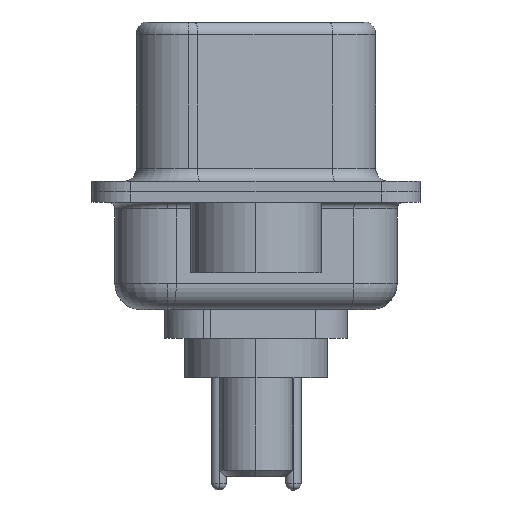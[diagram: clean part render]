
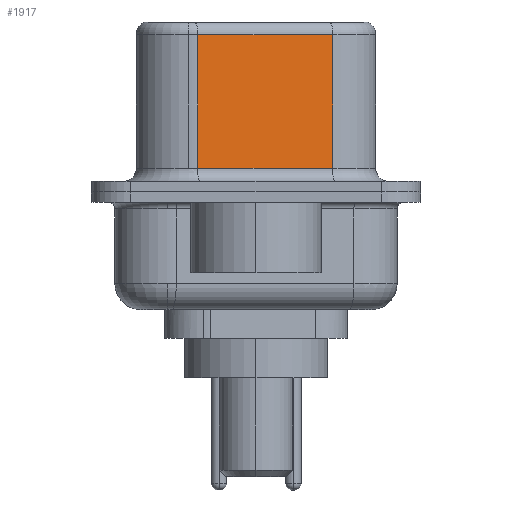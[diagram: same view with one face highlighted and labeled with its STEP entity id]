
A CAD part, left-side view. The second image highlights one B-rep face of the part: STEP entity #1917.
In plain terms, the highlighted planar face has unit normal (-0.985, -0.174, 0).
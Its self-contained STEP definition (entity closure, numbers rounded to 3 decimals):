
#178 = CARTESIAN_POINT ( 'NONE',  ( 3.675, 2.233, 6.52 ) ) ;
#355 = DIRECTION ( 'NONE',  ( -0.174, 0.985, 0. ) ) ;
#502 = CARTESIAN_POINT ( 'NONE',  ( 3.675, 2.233, 6.02 ) ) ;
#1160 = VECTOR ( 'NONE', #2051, 1000. ) ;
#1917 = ADVANCED_FACE ( 'NONE', ( #2913 ), #11902, .F. ) ;
#2051 = DIRECTION ( 'NONE',  ( 0., 0., -1. ) ) ;
#2913 = FACE_OUTER_BOUND ( 'NONE', #20003, .T. ) ;
#3100 = AXIS2_PLACEMENT_3D ( 'NONE', #11603, #4825, #8232 ) ;
#3354 = EDGE_CURVE ( 'NONE', #21944, #4846, #19706, .T. ) ;
#3679 = CARTESIAN_POINT ( 'NONE',  ( 4.585, -2.927, 6.02 ) ) ;
#3961 = LINE ( 'NONE', #21651, #10663 ) ;
#4825 = DIRECTION ( 'NONE',  ( 0.985, 0.174, 0. ) ) ;
#4846 = VERTEX_POINT ( 'NONE', #502 ) ;
#6582 = VECTOR ( 'NONE', #21888, 1000. ) ;
#8174 = LINE ( 'NONE', #20149, #6582 ) ;
#8232 = DIRECTION ( 'NONE',  ( -0.174, 0.985, 0. ) ) ;
#8790 = EDGE_CURVE ( 'NONE', #21944, #20865, #3961, .T. ) ;
#9247 = ORIENTED_EDGE ( 'NONE', *, *, #8790, .F. ) ;
#10112 = CARTESIAN_POINT ( 'NONE',  ( 3.675, 2.233, 0.9 ) ) ;
#10609 = EDGE_CURVE ( 'NONE', #12664, #20865, #8174, .T. ) ;
#10663 = VECTOR ( 'NONE', #19918, 1000. ) ;
#11603 = CARTESIAN_POINT ( 'NONE',  ( 4.585, -2.927, 6.52 ) ) ;
#11902 = PLANE ( 'NONE',  #3100 ) ;
#12664 = VERTEX_POINT ( 'NONE', #10112 ) ;
#12973 = ORIENTED_EDGE ( 'NONE', *, *, #10609, .T. ) ;
#13090 = CARTESIAN_POINT ( 'NONE',  ( 4.585, -2.927, 6.02 ) ) ;
#13882 = VECTOR ( 'NONE', #355, 1000. ) ;
#15932 = CARTESIAN_POINT ( 'NONE',  ( 4.585, -2.927, 0.9 ) ) ;
#18225 = ORIENTED_EDGE ( 'NONE', *, *, #20121, .T. ) ;
#18856 = ORIENTED_EDGE ( 'NONE', *, *, #3354, .T. ) ;
#19706 = LINE ( 'NONE', #3679, #13882 ) ;
#19918 = DIRECTION ( 'NONE',  ( 0., 0., -1. ) ) ;
#20003 = EDGE_LOOP ( 'NONE', ( #9247, #18856, #18225, #12973 ) ) ;
#20121 = EDGE_CURVE ( 'NONE', #4846, #12664, #21482, .T. ) ;
#20149 = CARTESIAN_POINT ( 'NONE',  ( 4.585, -2.927, 0.9 ) ) ;
#20865 = VERTEX_POINT ( 'NONE', #15932 ) ;
#21482 = LINE ( 'NONE', #178, #1160 ) ;
#21651 = CARTESIAN_POINT ( 'NONE',  ( 4.585, -2.927, 6.52 ) ) ;
#21888 = DIRECTION ( 'NONE',  ( 0.174, -0.985, 0. ) ) ;
#21944 = VERTEX_POINT ( 'NONE', #13090 ) ;
